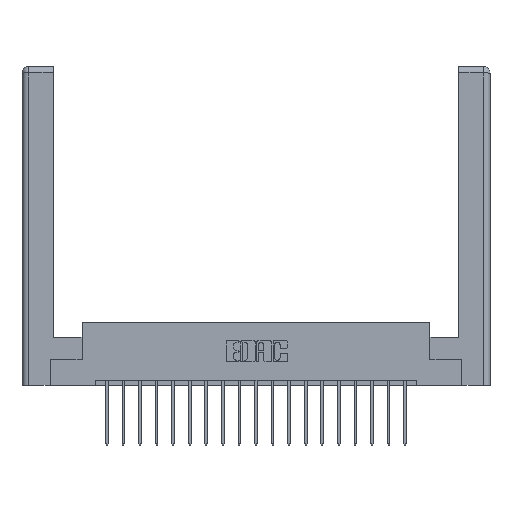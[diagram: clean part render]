
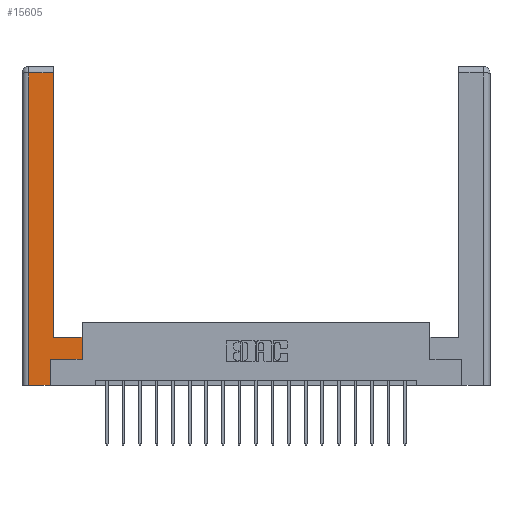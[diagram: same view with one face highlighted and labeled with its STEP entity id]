
A CAD part, top view. The second image highlights one B-rep face of the part: STEP entity #15605.
In plain terms, the highlighted planar face has unit normal (0, 0, 1).
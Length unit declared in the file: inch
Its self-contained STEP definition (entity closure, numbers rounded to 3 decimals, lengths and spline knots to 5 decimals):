
#70 = CARTESIAN_POINT ( 'NONE',  ( 0.265, 0., 0. ) ) ;
#288 = FACE_OUTER_BOUND ( 'NONE', #1965, .T. ) ;
#809 = LINE ( 'NONE', #14287, #12190 ) ;
#1965 = EDGE_LOOP ( 'NONE', ( #6246, #2517, #3626, #9976, #15924, #16708, #7753, #16113 ) ) ;
#1978 = EDGE_CURVE ( 'NONE', #2985, #15143, #18222, .T. ) ;
#2353 = LINE ( 'NONE', #4731, #14535 ) ;
#2517 = ORIENTED_EDGE ( 'NONE', *, *, #17092, .T. ) ;
#2736 = VECTOR ( 'NONE', #9510, 39.37008 ) ;
#2985 = VERTEX_POINT ( 'NONE', #16420 ) ;
#3162 = LINE ( 'NONE', #12644, #7575 ) ;
#3626 = ORIENTED_EDGE ( 'NONE', *, *, #17498, .T. ) ;
#4020 = LINE ( 'NONE', #8358, #12962 ) ;
#4346 = VERTEX_POINT ( 'NONE', #12347 ) ;
#4369 = EDGE_CURVE ( 'NONE', #14578, #13322, #13464, .T. ) ;
#4701 = DIRECTION ( 'NONE',  ( -1., 0., 0. ) ) ;
#4731 = CARTESIAN_POINT ( 'NONE',  ( 0.565, 0.245, 0. ) ) ;
#5266 = DIRECTION ( 'NONE',  ( 0., 1., 0. ) ) ;
#5701 = LINE ( 'NONE', #70, #2736 ) ;
#6089 = CARTESIAN_POINT ( 'NONE',  ( 0.265, 0.245, 0. ) ) ;
#6207 = DIRECTION ( 'NONE',  ( -1., 0., 0. ) ) ;
#6246 = ORIENTED_EDGE ( 'NONE', *, *, #4369, .T. ) ;
#6391 = DIRECTION ( 'NONE',  ( 0., 1., 0. ) ) ;
#6562 = VERTEX_POINT ( 'NONE', #13375 ) ;
#6647 = CARTESIAN_POINT ( 'NONE',  ( 0.295, 0.45, 0. ) ) ;
#7257 = VECTOR ( 'NONE', #6391, 39.37008 ) ;
#7575 = VECTOR ( 'NONE', #6207, 39.37008 ) ;
#7753 = ORIENTED_EDGE ( 'NONE', *, *, #8320, .T. ) ;
#7844 = PLANE ( 'NONE',  #19151 ) ;
#8320 = EDGE_CURVE ( 'NONE', #6562, #9721, #4020, .T. ) ;
#8358 = CARTESIAN_POINT ( 'NONE',  ( 0.565, 0.45, 0. ) ) ;
#9510 = DIRECTION ( 'NONE',  ( 1., 0., 0. ) ) ;
#9530 = DIRECTION ( 'NONE',  ( 0., 0., -1. ) ) ;
#9721 = VERTEX_POINT ( 'NONE', #19895 ) ;
#9976 = ORIENTED_EDGE ( 'NONE', *, *, #15226, .T. ) ;
#10862 = DIRECTION ( 'NONE',  ( -1., 0., 0. ) ) ;
#11209 = CARTESIAN_POINT ( 'NONE',  ( 0.0615, 2.94, 0. ) ) ;
#12190 = VECTOR ( 'NONE', #10862, 39.37008 ) ;
#12347 = CARTESIAN_POINT ( 'NONE',  ( 0.0615, 0., 0. ) ) ;
#12644 = CARTESIAN_POINT ( 'NONE',  ( 0.0615, 2.94, 0. ) ) ;
#12775 = CARTESIAN_POINT ( 'NONE',  ( 0.265, 0.245, 0. ) ) ;
#12962 = VECTOR ( 'NONE', #5266, 39.37008 ) ;
#12975 = DIRECTION ( 'NONE',  ( 0., -1., 0. ) ) ;
#13322 = VERTEX_POINT ( 'NONE', #15359 ) ;
#13375 = CARTESIAN_POINT ( 'NONE',  ( 0.565, 0.245, 0. ) ) ;
#13464 = LINE ( 'NONE', #15788, #7257 ) ;
#14287 = CARTESIAN_POINT ( 'NONE',  ( 0.295, 0.45, 0. ) ) ;
#14444 = DIRECTION ( 'NONE',  ( 1., 0., 0. ) ) ;
#14458 = DIRECTION ( 'NONE',  ( 0., 1., 0. ) ) ;
#14527 = EDGE_CURVE ( 'NONE', #9721, #14578, #809, .T. ) ;
#14535 = VECTOR ( 'NONE', #14444, 39.37008 ) ;
#14578 = VERTEX_POINT ( 'NONE', #6647 ) ;
#14583 = VERTEX_POINT ( 'NONE', #11209 ) ;
#14827 = VECTOR ( 'NONE', #14458, 39.37008 ) ;
#15143 = VERTEX_POINT ( 'NONE', #6089 ) ;
#15226 = EDGE_CURVE ( 'NONE', #4346, #2985, #5701, .T. ) ;
#15359 = CARTESIAN_POINT ( 'NONE',  ( 0.295, 2.94, 0. ) ) ;
#15605 = ADVANCED_FACE ( 'NONE', ( #288 ), #7844, .F. ) ;
#15788 = CARTESIAN_POINT ( 'NONE',  ( 0.295, 3., 0. ) ) ;
#15924 = ORIENTED_EDGE ( 'NONE', *, *, #1978, .T. ) ;
#16113 = ORIENTED_EDGE ( 'NONE', *, *, #14527, .T. ) ;
#16420 = CARTESIAN_POINT ( 'NONE',  ( 0.265, 0., 0. ) ) ;
#16500 = LINE ( 'NONE', #19330, #20141 ) ;
#16708 = ORIENTED_EDGE ( 'NONE', *, *, #19617, .T. ) ;
#17092 = EDGE_CURVE ( 'NONE', #13322, #14583, #3162, .T. ) ;
#17498 = EDGE_CURVE ( 'NONE', #14583, #4346, #16500, .T. ) ;
#18222 = LINE ( 'NONE', #12775, #14827 ) ;
#18900 = CARTESIAN_POINT ( 'NONE',  ( 0., 0., 0. ) ) ;
#19151 = AXIS2_PLACEMENT_3D ( 'NONE', #18900, #9530, #4701 ) ;
#19330 = CARTESIAN_POINT ( 'NONE',  ( 0.0615, 0., 0. ) ) ;
#19617 = EDGE_CURVE ( 'NONE', #15143, #6562, #2353, .T. ) ;
#19895 = CARTESIAN_POINT ( 'NONE',  ( 0.565, 0.45, 0. ) ) ;
#20141 = VECTOR ( 'NONE', #12975, 39.37008 ) ;
